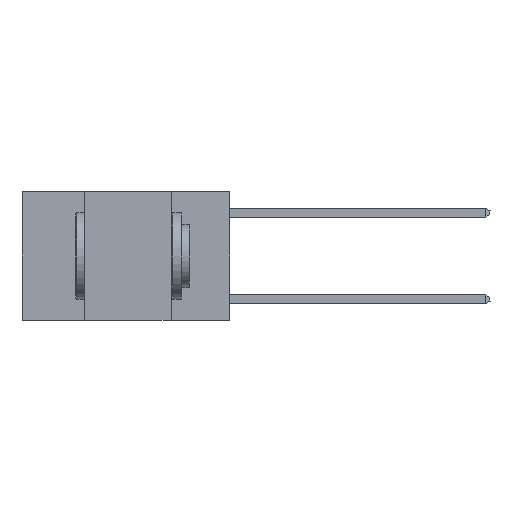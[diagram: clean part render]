
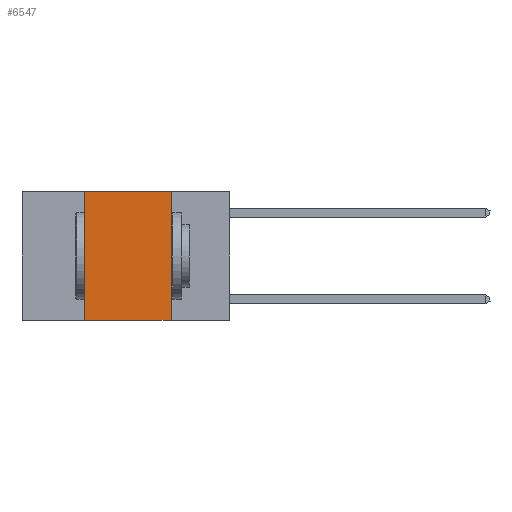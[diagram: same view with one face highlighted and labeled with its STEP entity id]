
A CAD part, left-side view. The second image highlights one B-rep face of the part: STEP entity #6547.
In plain terms, the highlighted planar face has unit normal (-1, 0, 0).
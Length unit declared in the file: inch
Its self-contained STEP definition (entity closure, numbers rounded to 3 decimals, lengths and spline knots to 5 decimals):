
#228 = DIRECTION ( 'NONE',  ( 0., 0., -1. ) ) ;
#444 = CARTESIAN_POINT ( 'NONE',  ( 0., 0.42, -0.37 ) ) ;
#637 = VERTEX_POINT ( 'NONE', #7664 ) ;
#3179 = CARTESIAN_POINT ( 'NONE',  ( 0., 0.17, 0. ) ) ;
#3710 = ORIENTED_EDGE ( 'NONE', *, *, #17611, .F. ) ;
#4949 = AXIS2_PLACEMENT_3D ( 'NONE', #10698, #19274, #6998 ) ;
#5871 = VECTOR ( 'NONE', #6182, 39.37008 ) ;
#6182 = DIRECTION ( 'NONE',  ( 0., -1., 0. ) ) ;
#6547 = ADVANCED_FACE ( 'NONE', ( #19166 ), #17768, .F. ) ;
#6704 = CARTESIAN_POINT ( 'NONE',  ( 0., 0.42, 0. ) ) ;
#6998 = DIRECTION ( 'NONE',  ( 0., 0., -1. ) ) ;
#7131 = DIRECTION ( 'NONE',  ( 0., -1., 0. ) ) ;
#7559 = LINE ( 'NONE', #16364, #19843 ) ;
#7664 = CARTESIAN_POINT ( 'NONE',  ( 0., 0.17, -0.37 ) ) ;
#7983 = EDGE_LOOP ( 'NONE', ( #12295, #17134, #3710, #14376 ) ) ;
#9769 = LINE ( 'NONE', #22077, #5871 ) ;
#10527 = DIRECTION ( 'NONE',  ( 0., 0., 1. ) ) ;
#10614 = CARTESIAN_POINT ( 'NONE',  ( 0., 0.6, -0.37 ) ) ;
#10698 = CARTESIAN_POINT ( 'NONE',  ( 0., 0.6, 0. ) ) ;
#10831 = LINE ( 'NONE', #10614, #10953 ) ;
#10953 = VECTOR ( 'NONE', #7131, 39.37008 ) ;
#12295 = ORIENTED_EDGE ( 'NONE', *, *, #15484, .F. ) ;
#14276 = VERTEX_POINT ( 'NONE', #19459 ) ;
#14306 = VECTOR ( 'NONE', #10527, 39.37008 ) ;
#14376 = ORIENTED_EDGE ( 'NONE', *, *, #16789, .T. ) ;
#15484 = EDGE_CURVE ( 'NONE', #22621, #637, #7559, .T. ) ;
#16364 = CARTESIAN_POINT ( 'NONE',  ( 0., 0.17, 0. ) ) ;
#16789 = EDGE_CURVE ( 'NONE', #21476, #637, #10831, .T. ) ;
#17134 = ORIENTED_EDGE ( 'NONE', *, *, #19869, .F. ) ;
#17611 = EDGE_CURVE ( 'NONE', #21476, #14276, #19446, .T. ) ;
#17768 = PLANE ( 'NONE',  #4949 ) ;
#19166 = FACE_OUTER_BOUND ( 'NONE', #7983, .T. ) ;
#19274 = DIRECTION ( 'NONE',  ( 1., 0., 0. ) ) ;
#19446 = LINE ( 'NONE', #6704, #14306 ) ;
#19459 = CARTESIAN_POINT ( 'NONE',  ( 0., 0.42, 0. ) ) ;
#19843 = VECTOR ( 'NONE', #228, 39.37008 ) ;
#19869 = EDGE_CURVE ( 'NONE', #14276, #22621, #9769, .T. ) ;
#21476 = VERTEX_POINT ( 'NONE', #444 ) ;
#22077 = CARTESIAN_POINT ( 'NONE',  ( 0., 0.6, 0. ) ) ;
#22621 = VERTEX_POINT ( 'NONE', #3179 ) ;
